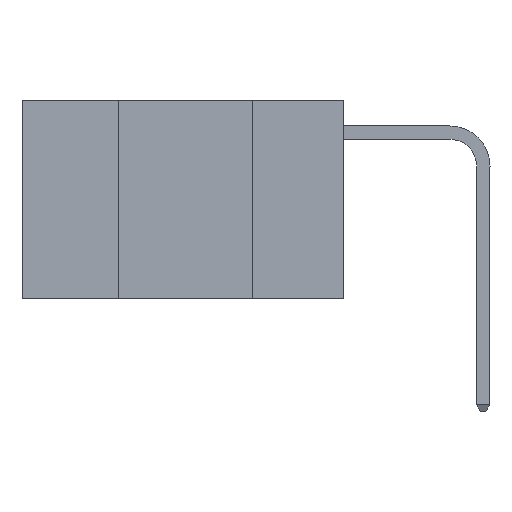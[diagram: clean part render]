
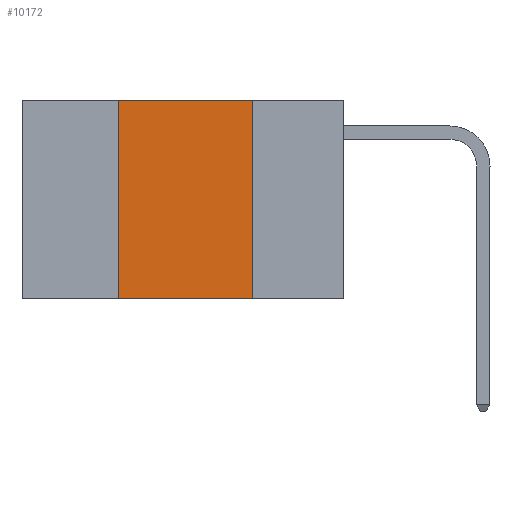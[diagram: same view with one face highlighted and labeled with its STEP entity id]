
A CAD part, left-side view. The second image highlights one B-rep face of the part: STEP entity #10172.
In plain terms, the highlighted planar face has unit normal (-1, 0, 0).
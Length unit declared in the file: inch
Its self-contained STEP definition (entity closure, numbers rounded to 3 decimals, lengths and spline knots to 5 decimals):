
#361 = VERTEX_POINT ( 'NONE', #5910 ) ;
#676 = FACE_OUTER_BOUND ( 'NONE', #10423, .T. ) ;
#905 = LINE ( 'NONE', #7340, #9019 ) ;
#1277 = PLANE ( 'NONE',  #8554 ) ;
#1614 = DIRECTION ( 'NONE',  ( 0., -1., 0. ) ) ;
#1957 = LINE ( 'NONE', #2284, #6066 ) ;
#2284 = CARTESIAN_POINT ( 'NONE',  ( 0., 0.6, 0. ) ) ;
#2941 = DIRECTION ( 'NONE',  ( 0., 0., -1. ) ) ;
#3110 = CARTESIAN_POINT ( 'NONE',  ( 0., 0.42, 0. ) ) ;
#3114 = DIRECTION ( 'NONE',  ( 0., -1., 0. ) ) ;
#3407 = VERTEX_POINT ( 'NONE', #5489 ) ;
#3795 = VECTOR ( 'NONE', #1614, 39.37008 ) ;
#4077 = VERTEX_POINT ( 'NONE', #3110 ) ;
#4551 = ORIENTED_EDGE ( 'NONE', *, *, #7493, .F. ) ;
#4613 = ORIENTED_EDGE ( 'NONE', *, *, #7369, .F. ) ;
#4694 = LINE ( 'NONE', #8063, #8450 ) ;
#4712 = ORIENTED_EDGE ( 'NONE', *, *, #10393, .F. ) ;
#5199 = CARTESIAN_POINT ( 'NONE',  ( 0., 0.17, -0.37 ) ) ;
#5489 = CARTESIAN_POINT ( 'NONE',  ( 0., 0.42, -0.37 ) ) ;
#5599 = ORIENTED_EDGE ( 'NONE', *, *, #9821, .T. ) ;
#5910 = CARTESIAN_POINT ( 'NONE',  ( 0., 0.17, 0. ) ) ;
#6066 = VECTOR ( 'NONE', #3114, 39.37008 ) ;
#6226 = LINE ( 'NONE', #9663, #3795 ) ;
#7007 = CARTESIAN_POINT ( 'NONE',  ( 0., 0.6, 0. ) ) ;
#7340 = CARTESIAN_POINT ( 'NONE',  ( 0., 0.17, 0. ) ) ;
#7369 = EDGE_CURVE ( 'NONE', #4077, #361, #1957, .T. ) ;
#7493 = EDGE_CURVE ( 'NONE', #361, #8856, #905, .T. ) ;
#7793 = DIRECTION ( 'NONE',  ( 1., 0., 0. ) ) ;
#8063 = CARTESIAN_POINT ( 'NONE',  ( 0., 0.42, 0. ) ) ;
#8126 = DIRECTION ( 'NONE',  ( 0., 0., -1. ) ) ;
#8450 = VECTOR ( 'NONE', #9649, 39.37008 ) ;
#8554 = AXIS2_PLACEMENT_3D ( 'NONE', #7007, #7793, #2941 ) ;
#8856 = VERTEX_POINT ( 'NONE', #5199 ) ;
#9019 = VECTOR ( 'NONE', #8126, 39.37008 ) ;
#9649 = DIRECTION ( 'NONE',  ( 0., 0., 1. ) ) ;
#9663 = CARTESIAN_POINT ( 'NONE',  ( 0., 0.6, -0.37 ) ) ;
#9821 = EDGE_CURVE ( 'NONE', #3407, #8856, #6226, .T. ) ;
#10172 = ADVANCED_FACE ( 'NONE', ( #676 ), #1277, .F. ) ;
#10393 = EDGE_CURVE ( 'NONE', #3407, #4077, #4694, .T. ) ;
#10423 = EDGE_LOOP ( 'NONE', ( #4551, #4613, #4712, #5599 ) ) ;
